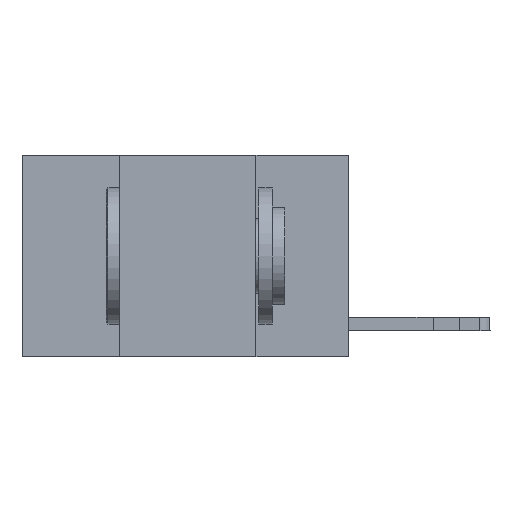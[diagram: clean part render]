
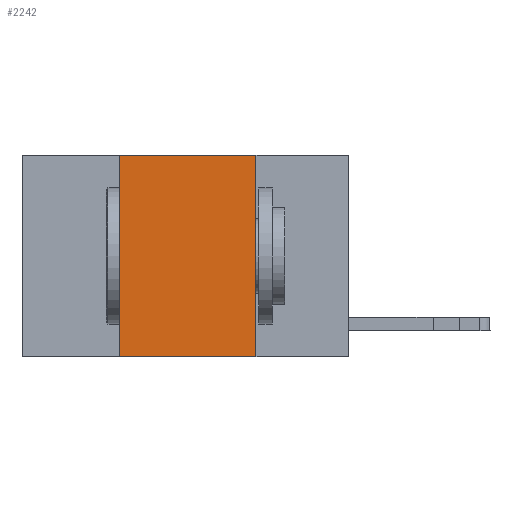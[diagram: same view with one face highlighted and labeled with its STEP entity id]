
A CAD part, left-side view. The second image highlights one B-rep face of the part: STEP entity #2242.
In plain terms, the highlighted planar face has unit normal (-1, 0, 0).
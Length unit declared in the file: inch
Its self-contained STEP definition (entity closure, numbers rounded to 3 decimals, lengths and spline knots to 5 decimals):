
#32 = ORIENTED_EDGE ( 'NONE', *, *, #10036, .F. ) ;
#195 = FACE_OUTER_BOUND ( 'NONE', #353, .T. ) ;
#353 = EDGE_LOOP ( 'NONE', ( #19840, #32, #2360, #26045 ) ) ;
#1331 = CARTESIAN_POINT ( 'NONE',  ( 0., 0.42, -0.37 ) ) ;
#2242 = ADVANCED_FACE ( 'NONE', ( #195 ), #9125, .F. ) ;
#2335 = VECTOR ( 'NONE', #25467, 39.37008 ) ;
#2360 = ORIENTED_EDGE ( 'NONE', *, *, #3642, .F. ) ;
#2753 = VERTEX_POINT ( 'NONE', #2993 ) ;
#2993 = CARTESIAN_POINT ( 'NONE',  ( 0., 0.42, 0. ) ) ;
#3612 = CARTESIAN_POINT ( 'NONE',  ( 0., 0.42, 0. ) ) ;
#3642 = EDGE_CURVE ( 'NONE', #16704, #2753, #18074, .T. ) ;
#4176 = LINE ( 'NONE', #12572, #22546 ) ;
#4833 = VECTOR ( 'NONE', #12011, 39.37008 ) ;
#8657 = CARTESIAN_POINT ( 'NONE',  ( 0., 0.17, 0. ) ) ;
#8715 = DIRECTION ( 'NONE',  ( 0., -1., 0. ) ) ;
#9125 = PLANE ( 'NONE',  #24583 ) ;
#10036 = EDGE_CURVE ( 'NONE', #2753, #20095, #15927, .T. ) ;
#12011 = DIRECTION ( 'NONE',  ( 0., 0., 1. ) ) ;
#12068 = DIRECTION ( 'NONE',  ( 0., -1., 0. ) ) ;
#12572 = CARTESIAN_POINT ( 'NONE',  ( 0., 0.6, -0.37 ) ) ;
#12913 = VERTEX_POINT ( 'NONE', #15349 ) ;
#15349 = CARTESIAN_POINT ( 'NONE',  ( 0., 0.17, -0.37 ) ) ;
#15927 = LINE ( 'NONE', #24745, #22862 ) ;
#16704 = VERTEX_POINT ( 'NONE', #1331 ) ;
#18074 = LINE ( 'NONE', #3612, #4833 ) ;
#19840 = ORIENTED_EDGE ( 'NONE', *, *, #21331, .F. ) ;
#20095 = VERTEX_POINT ( 'NONE', #22132 ) ;
#21331 = EDGE_CURVE ( 'NONE', #20095, #12913, #21464, .T. ) ;
#21394 = DIRECTION ( 'NONE',  ( 1., 0., 0. ) ) ;
#21464 = LINE ( 'NONE', #8657, #2335 ) ;
#22132 = CARTESIAN_POINT ( 'NONE',  ( 0., 0.17, 0. ) ) ;
#22546 = VECTOR ( 'NONE', #8715, 39.37008 ) ;
#22862 = VECTOR ( 'NONE', #12068, 39.37008 ) ;
#23164 = EDGE_CURVE ( 'NONE', #16704, #12913, #4176, .T. ) ;
#24583 = AXIS2_PLACEMENT_3D ( 'NONE', #25788, #21394, #25660 ) ;
#24745 = CARTESIAN_POINT ( 'NONE',  ( 0., 0.6, 0. ) ) ;
#25467 = DIRECTION ( 'NONE',  ( 0., 0., -1. ) ) ;
#25660 = DIRECTION ( 'NONE',  ( 0., 0., -1. ) ) ;
#25788 = CARTESIAN_POINT ( 'NONE',  ( 0., 0.6, 0. ) ) ;
#26045 = ORIENTED_EDGE ( 'NONE', *, *, #23164, .T. ) ;
